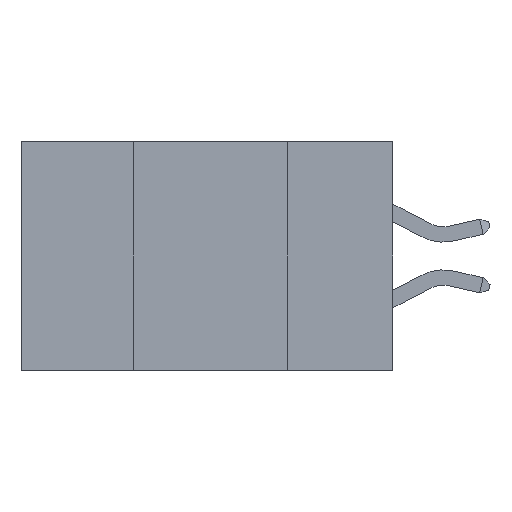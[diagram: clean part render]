
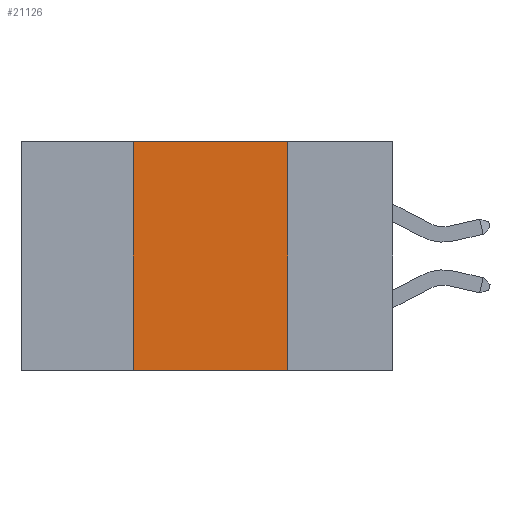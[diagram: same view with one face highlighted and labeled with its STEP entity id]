
A CAD part, left-side view. The second image highlights one B-rep face of the part: STEP entity #21126.
In plain terms, the highlighted planar face has unit normal (-1, 0, 0).
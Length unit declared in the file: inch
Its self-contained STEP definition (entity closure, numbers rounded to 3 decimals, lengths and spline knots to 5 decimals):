
#1201 = CARTESIAN_POINT ( 'NONE',  ( 0., 0.17, -0.37 ) ) ;
#1419 = ORIENTED_EDGE ( 'NONE', *, *, #6855, .F. ) ;
#1510 = VERTEX_POINT ( 'NONE', #1201 ) ;
#1886 = VERTEX_POINT ( 'NONE', #2203 ) ;
#2129 = ORIENTED_EDGE ( 'NONE', *, *, #15913, .T. ) ;
#2203 = CARTESIAN_POINT ( 'NONE',  ( 0., 0.42, -0.37 ) ) ;
#4266 = VERTEX_POINT ( 'NONE', #8179 ) ;
#4482 = LINE ( 'NONE', #10155, #18694 ) ;
#4532 = EDGE_LOOP ( 'NONE', ( #23387, #1419, #21938, #2129 ) ) ;
#4621 = CARTESIAN_POINT ( 'NONE',  ( 0., 0.17, 0. ) ) ;
#4976 = VERTEX_POINT ( 'NONE', #4621 ) ;
#5181 = FACE_OUTER_BOUND ( 'NONE', #4532, .T. ) ;
#6043 = VECTOR ( 'NONE', #21877, 39.37008 ) ;
#6076 = AXIS2_PLACEMENT_3D ( 'NONE', #21315, #23170, #12161 ) ;
#6427 = DIRECTION ( 'NONE',  ( 0., -1., 0. ) ) ;
#6501 = CARTESIAN_POINT ( 'NONE',  ( 0., 0.42, 0. ) ) ;
#6855 = EDGE_CURVE ( 'NONE', #4266, #4976, #4482, .T. ) ;
#8179 = CARTESIAN_POINT ( 'NONE',  ( 0., 0.42, 0. ) ) ;
#8448 = PLANE ( 'NONE',  #6076 ) ;
#10155 = CARTESIAN_POINT ( 'NONE',  ( 0., 0.6, 0. ) ) ;
#10834 = CARTESIAN_POINT ( 'NONE',  ( 0., 0.6, -0.37 ) ) ;
#11008 = LINE ( 'NONE', #10834, #6043 ) ;
#12161 = DIRECTION ( 'NONE',  ( 0., 0., -1. ) ) ;
#14415 = CARTESIAN_POINT ( 'NONE',  ( 0., 0.17, 0. ) ) ;
#14509 = LINE ( 'NONE', #14415, #15079 ) ;
#14707 = EDGE_CURVE ( 'NONE', #4976, #1510, #14509, .T. ) ;
#15079 = VECTOR ( 'NONE', #19968, 39.37008 ) ;
#15145 = EDGE_CURVE ( 'NONE', #1886, #4266, #22568, .T. ) ;
#15913 = EDGE_CURVE ( 'NONE', #1886, #1510, #11008, .T. ) ;
#17527 = DIRECTION ( 'NONE',  ( 0., 0., 1. ) ) ;
#17659 = VECTOR ( 'NONE', #17527, 39.37008 ) ;
#18694 = VECTOR ( 'NONE', #6427, 39.37008 ) ;
#19968 = DIRECTION ( 'NONE',  ( 0., 0., -1. ) ) ;
#21126 = ADVANCED_FACE ( 'NONE', ( #5181 ), #8448, .F. ) ;
#21315 = CARTESIAN_POINT ( 'NONE',  ( 0., 0.6, 0. ) ) ;
#21877 = DIRECTION ( 'NONE',  ( 0., -1., 0. ) ) ;
#21938 = ORIENTED_EDGE ( 'NONE', *, *, #15145, .F. ) ;
#22568 = LINE ( 'NONE', #6501, #17659 ) ;
#23170 = DIRECTION ( 'NONE',  ( 1., 0., 0. ) ) ;
#23387 = ORIENTED_EDGE ( 'NONE', *, *, #14707, .F. ) ;
